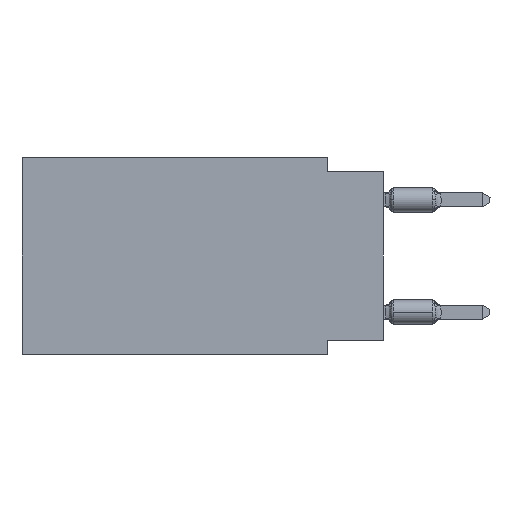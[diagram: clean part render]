
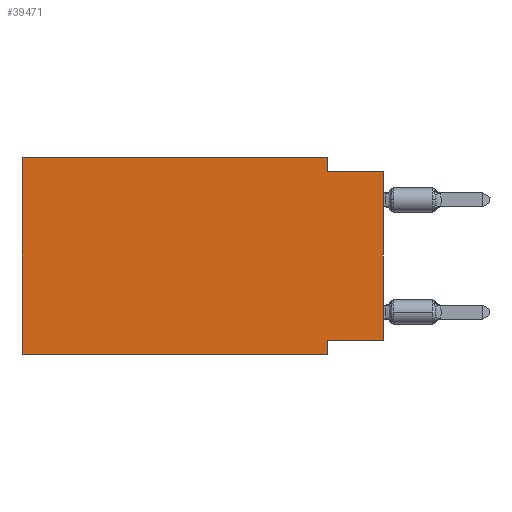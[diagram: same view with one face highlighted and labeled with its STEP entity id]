
A CAD part, left-side view. The second image highlights one B-rep face of the part: STEP entity #39471.
In plain terms, the highlighted planar face has unit normal (-1, 0, 0).
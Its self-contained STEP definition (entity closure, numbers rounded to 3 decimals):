
#639 = VERTEX_POINT ( 'NONE', #19685 ) ;
#2975 = EDGE_CURVE ( 'NONE', #42408, #4491, #35241, .T. ) ;
#3175 = DIRECTION ( 'NONE',  ( 0., -1., 0. ) ) ;
#3730 = AXIS2_PLACEMENT_3D ( 'NONE', #8769, #3799, #31078 ) ;
#3799 = DIRECTION ( 'NONE',  ( 1., 0., 0. ) ) ;
#4483 = VECTOR ( 'NONE', #19716, 1000. ) ;
#4491 = VERTEX_POINT ( 'NONE', #27276 ) ;
#4774 = VECTOR ( 'NONE', #46698, 1000. ) ;
#5688 = CARTESIAN_POINT ( 'NONE',  ( 0., 2.54, -8.89 ) ) ;
#6365 = LINE ( 'NONE', #21509, #42041 ) ;
#6422 = DIRECTION ( 'NONE',  ( 0., 0., -1. ) ) ;
#6470 = VERTEX_POINT ( 'NONE', #5688 ) ;
#7937 = VECTOR ( 'NONE', #3175, 1000. ) ;
#8551 = LINE ( 'NONE', #39299, #4483 ) ;
#8769 = CARTESIAN_POINT ( 'NONE',  ( 0., 16.383, 0. ) ) ;
#9352 = DIRECTION ( 'NONE',  ( 0., 1., 0. ) ) ;
#10006 = ORIENTED_EDGE ( 'NONE', *, *, #15653, .T. ) ;
#11732 = ORIENTED_EDGE ( 'NONE', *, *, #12314, .F. ) ;
#11742 = VERTEX_POINT ( 'NONE', #36492 ) ;
#12097 = CARTESIAN_POINT ( 'NONE',  ( 0., 0., -8.255 ) ) ;
#12314 = EDGE_CURVE ( 'NONE', #639, #11742, #37166, .T. ) ;
#12419 = EDGE_LOOP ( 'NONE', ( #38468, #11732, #39128, #20412, #48491, #10006, #48057, #43638 ) ) ;
#12606 = EDGE_CURVE ( 'NONE', #47964, #6470, #6365, .T. ) ;
#14584 = CARTESIAN_POINT ( 'NONE',  ( 0., 0., -0.635 ) ) ;
#15653 = EDGE_CURVE ( 'NONE', #42408, #6470, #35734, .T. ) ;
#16886 = DIRECTION ( 'NONE',  ( 0., -1., 0. ) ) ;
#16907 = CARTESIAN_POINT ( 'NONE',  ( 0., 16.383, 0. ) ) ;
#17483 = EDGE_CURVE ( 'NONE', #26871, #639, #29235, .T. ) ;
#19286 = EDGE_CURVE ( 'NONE', #43684, #11742, #8551, .T. ) ;
#19685 = CARTESIAN_POINT ( 'NONE',  ( 0., 2.54, -0.635 ) ) ;
#19716 = DIRECTION ( 'NONE',  ( 0., 0., 1. ) ) ;
#20412 = ORIENTED_EDGE ( 'NONE', *, *, #38804, .F. ) ;
#20758 = DIRECTION ( 'NONE',  ( 0., 0., -1. ) ) ;
#21143 = VECTOR ( 'NONE', #9352, 1000. ) ;
#21509 = CARTESIAN_POINT ( 'NONE',  ( 0., 2.54, -8.89 ) ) ;
#23491 = CARTESIAN_POINT ( 'NONE',  ( 0., 16.383, -8.89 ) ) ;
#23737 = CARTESIAN_POINT ( 'NONE',  ( 0., 0., -8.255 ) ) ;
#25113 = EDGE_CURVE ( 'NONE', #43684, #47964, #46557, .T. ) ;
#26617 = PLANE ( 'NONE',  #3730 ) ;
#26871 = VERTEX_POINT ( 'NONE', #32341 ) ;
#27115 = FACE_OUTER_BOUND ( 'NONE', #12419, .T. ) ;
#27276 = CARTESIAN_POINT ( 'NONE',  ( 0., 16.383, 0. ) ) ;
#27542 = CARTESIAN_POINT ( 'NONE',  ( 0., 16.383, 0. ) ) ;
#29235 = LINE ( 'NONE', #47857, #39263 ) ;
#31078 = DIRECTION ( 'NONE',  ( 0., 0., -1. ) ) ;
#31757 = LINE ( 'NONE', #27542, #44890 ) ;
#32341 = CARTESIAN_POINT ( 'NONE',  ( 0., 2.54, 0. ) ) ;
#35241 = LINE ( 'NONE', #16907, #4774 ) ;
#35734 = LINE ( 'NONE', #39701, #44966 ) ;
#36492 = CARTESIAN_POINT ( 'NONE',  ( 0., 0., -0.635 ) ) ;
#37166 = LINE ( 'NONE', #14584, #7937 ) ;
#38468 = ORIENTED_EDGE ( 'NONE', *, *, #19286, .T. ) ;
#38804 = EDGE_CURVE ( 'NONE', #4491, #26871, #31757, .T. ) ;
#39128 = ORIENTED_EDGE ( 'NONE', *, *, #17483, .F. ) ;
#39263 = VECTOR ( 'NONE', #6422, 1000. ) ;
#39299 = CARTESIAN_POINT ( 'NONE',  ( 0., 0., 0. ) ) ;
#39471 = ADVANCED_FACE ( 'NONE', ( #27115 ), #26617, .F. ) ;
#39701 = CARTESIAN_POINT ( 'NONE',  ( 0., 16.383, -8.89 ) ) ;
#42041 = VECTOR ( 'NONE', #20758, 1000. ) ;
#42408 = VERTEX_POINT ( 'NONE', #23491 ) ;
#43638 = ORIENTED_EDGE ( 'NONE', *, *, #25113, .F. ) ;
#43684 = VERTEX_POINT ( 'NONE', #12097 ) ;
#44890 = VECTOR ( 'NONE', #46909, 1000. ) ;
#44966 = VECTOR ( 'NONE', #16886, 1000. ) ;
#46557 = LINE ( 'NONE', #23737, #21143 ) ;
#46698 = DIRECTION ( 'NONE',  ( 0., 0., 1. ) ) ;
#46909 = DIRECTION ( 'NONE',  ( 0., -1., 0. ) ) ;
#47857 = CARTESIAN_POINT ( 'NONE',  ( 0., 2.54, 0. ) ) ;
#47964 = VERTEX_POINT ( 'NONE', #48723 ) ;
#48057 = ORIENTED_EDGE ( 'NONE', *, *, #12606, .F. ) ;
#48491 = ORIENTED_EDGE ( 'NONE', *, *, #2975, .F. ) ;
#48723 = CARTESIAN_POINT ( 'NONE',  ( 0., 2.54, -8.255 ) ) ;
